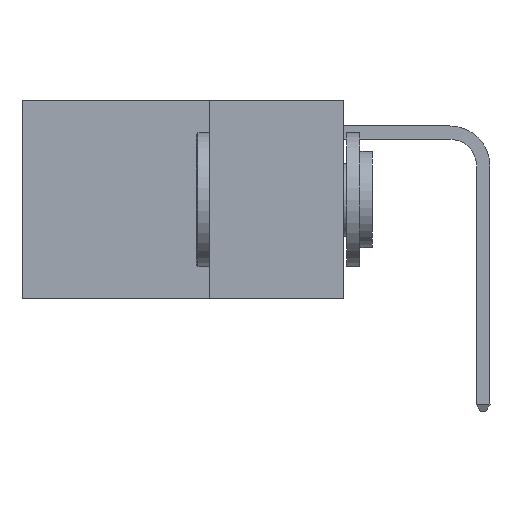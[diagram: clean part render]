
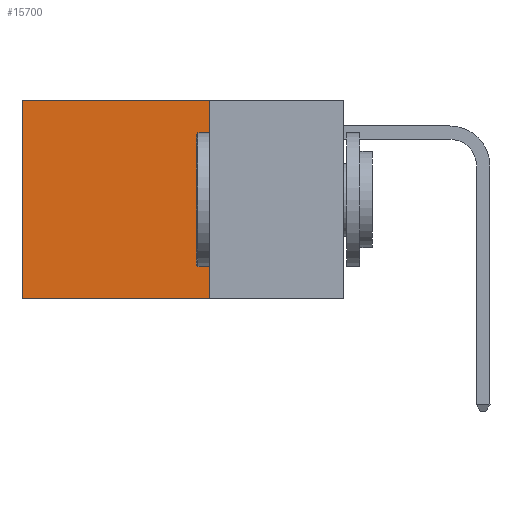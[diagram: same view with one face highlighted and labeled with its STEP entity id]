
A CAD part, left-side view. The second image highlights one B-rep face of the part: STEP entity #15700.
In plain terms, the highlighted planar face has unit normal (-1, 0, 0).
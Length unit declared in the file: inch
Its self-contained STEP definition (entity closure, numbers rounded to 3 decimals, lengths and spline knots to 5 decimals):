
#789 = CARTESIAN_POINT ( 'NONE',  ( 0.2625, 0.6, 0. ) ) ;
#1014 = EDGE_LOOP ( 'NONE', ( #16285, #10307, #3012, #1580 ) ) ;
#1580 = ORIENTED_EDGE ( 'NONE', *, *, #13466, .T. ) ;
#1618 = LINE ( 'NONE', #16030, #12853 ) ;
#1628 = DIRECTION ( 'NONE',  ( 0., 1., 0. ) ) ;
#2322 = CARTESIAN_POINT ( 'NONE',  ( 0.2625, 0.6, -0.37 ) ) ;
#3012 = ORIENTED_EDGE ( 'NONE', *, *, #6743, .F. ) ;
#3311 = VERTEX_POINT ( 'NONE', #3606 ) ;
#3606 = CARTESIAN_POINT ( 'NONE',  ( 0.2625, 0.25, 0. ) ) ;
#3608 = VECTOR ( 'NONE', #1628, 39.37008 ) ;
#3642 = VERTEX_POINT ( 'NONE', #2322 ) ;
#3788 = CARTESIAN_POINT ( 'NONE',  ( 0.2625, 0.25, 0. ) ) ;
#6232 = FACE_OUTER_BOUND ( 'NONE', #1014, .T. ) ;
#6743 = EDGE_CURVE ( 'NONE', #3311, #8852, #7769, .T. ) ;
#7419 = AXIS2_PLACEMENT_3D ( 'NONE', #3788, #15780, #8878 ) ;
#7691 = DIRECTION ( 'NONE',  ( 0., 0., -1. ) ) ;
#7722 = EDGE_CURVE ( 'NONE', #15678, #3642, #1618, .T. ) ;
#7769 = LINE ( 'NONE', #16085, #12685 ) ;
#8046 = LINE ( 'NONE', #13418, #8663 ) ;
#8663 = VECTOR ( 'NONE', #9448, 39.37008 ) ;
#8852 = VERTEX_POINT ( 'NONE', #16935 ) ;
#8878 = DIRECTION ( 'NONE',  ( 0., 0., -1. ) ) ;
#9448 = DIRECTION ( 'NONE',  ( 0., 1., 0. ) ) ;
#10307 = ORIENTED_EDGE ( 'NONE', *, *, #10823, .F. ) ;
#10823 = EDGE_CURVE ( 'NONE', #8852, #3642, #8046, .T. ) ;
#11838 = PLANE ( 'NONE',  #7419 ) ;
#12239 = CARTESIAN_POINT ( 'NONE',  ( 0.2625, 0.25, 0. ) ) ;
#12401 = DIRECTION ( 'NONE',  ( 0., 0., -1. ) ) ;
#12417 = LINE ( 'NONE', #12239, #3608 ) ;
#12685 = VECTOR ( 'NONE', #7691, 39.37008 ) ;
#12853 = VECTOR ( 'NONE', #12401, 39.37008 ) ;
#13418 = CARTESIAN_POINT ( 'NONE',  ( 0.2625, 0.25, -0.37 ) ) ;
#13466 = EDGE_CURVE ( 'NONE', #3311, #15678, #12417, .T. ) ;
#15678 = VERTEX_POINT ( 'NONE', #789 ) ;
#15700 = ADVANCED_FACE ( 'NONE', ( #6232 ), #11838, .F. ) ;
#15780 = DIRECTION ( 'NONE',  ( 1., 0., 0. ) ) ;
#16030 = CARTESIAN_POINT ( 'NONE',  ( 0.2625, 0.6, 0. ) ) ;
#16085 = CARTESIAN_POINT ( 'NONE',  ( 0.2625, 0.25, 0. ) ) ;
#16285 = ORIENTED_EDGE ( 'NONE', *, *, #7722, .T. ) ;
#16935 = CARTESIAN_POINT ( 'NONE',  ( 0.2625, 0.25, -0.37 ) ) ;
